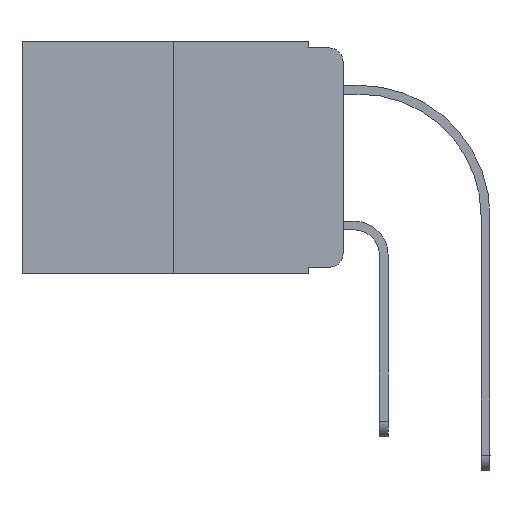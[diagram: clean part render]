
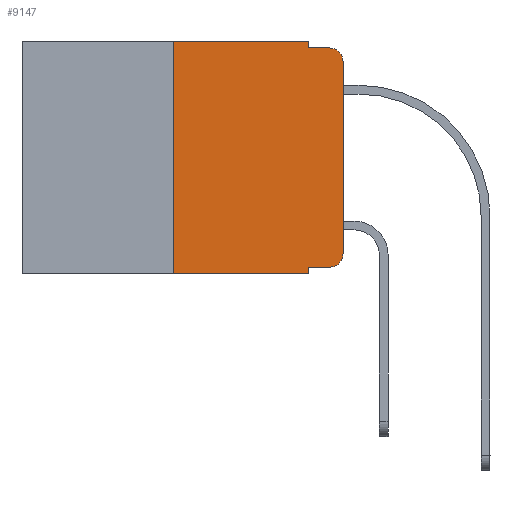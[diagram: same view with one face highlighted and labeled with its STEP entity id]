
A CAD part, left-side view. The second image highlights one B-rep face of the part: STEP entity #9147.
In plain terms, the highlighted planar face has unit normal (-1, 0, 0).
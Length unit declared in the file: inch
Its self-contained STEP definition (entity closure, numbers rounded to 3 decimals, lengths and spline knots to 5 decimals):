
#3 = DIRECTION ( 'NONE',  ( 0., 0., -1. ) ) ;
#83 = FACE_OUTER_BOUND ( 'NONE', #6889, .T. ) ;
#214 = CARTESIAN_POINT ( 'NONE',  ( 0., 0., -0.313 ) ) ;
#323 = ORIENTED_EDGE ( 'NONE', *, *, #11098, .T. ) ;
#342 = VERTEX_POINT ( 'NONE', #9852 ) ;
#380 = VERTEX_POINT ( 'NONE', #2476 ) ;
#1178 = CARTESIAN_POINT ( 'NONE',  ( 0., 0.051, 0. ) ) ;
#1305 = ORIENTED_EDGE ( 'NONE', *, *, #3405, .T. ) ;
#1357 = CARTESIAN_POINT ( 'NONE',  ( 0., 0.051, -0.01 ) ) ;
#2319 = CIRCLE ( 'NONE', #10659, 0.02 ) ;
#2476 = CARTESIAN_POINT ( 'NONE',  ( 0., 0., -0.03 ) ) ;
#2523 = DIRECTION ( 'NONE',  ( 0., -1., 0. ) ) ;
#2785 = VERTEX_POINT ( 'NONE', #7133 ) ;
#2890 = ORIENTED_EDGE ( 'NONE', *, *, #10798, .T. ) ;
#3113 = CARTESIAN_POINT ( 'NONE',  ( 0., 0.051, -0.333 ) ) ;
#3405 = EDGE_CURVE ( 'NONE', #9787, #10544, #13211, .T. ) ;
#3697 = VECTOR ( 'NONE', #7472, 39.37008 ) ;
#3719 = VECTOR ( 'NONE', #14480, 39.37008 ) ;
#3730 = VERTEX_POINT ( 'NONE', #1357 ) ;
#4233 = VECTOR ( 'NONE', #2523, 39.37008 ) ;
#4420 = ORIENTED_EDGE ( 'NONE', *, *, #8532, .F. ) ;
#4503 = EDGE_CURVE ( 'NONE', #342, #10544, #4986, .T. ) ;
#4505 = EDGE_CURVE ( 'NONE', #6124, #380, #13257, .T. ) ;
#4549 = VERTEX_POINT ( 'NONE', #7572 ) ;
#4603 = CARTESIAN_POINT ( 'NONE',  ( 0., 0.473, 0. ) ) ;
#4986 = LINE ( 'NONE', #9530, #6417 ) ;
#5717 = DIRECTION ( 'NONE',  ( -1., 0., 0. ) ) ;
#5748 = DIRECTION ( 'NONE',  ( 0., 0., -1. ) ) ;
#6090 = ORIENTED_EDGE ( 'NONE', *, *, #10879, .F. ) ;
#6124 = VERTEX_POINT ( 'NONE', #214 ) ;
#6183 = CARTESIAN_POINT ( 'NONE',  ( 0., 0.473, -0.343 ) ) ;
#6202 = DIRECTION ( 'NONE',  ( -1., 0., 0. ) ) ;
#6411 = CARTESIAN_POINT ( 'NONE',  ( 0., 0.051, -0.01 ) ) ;
#6417 = VECTOR ( 'NONE', #8397, 39.37008 ) ;
#6694 = PLANE ( 'NONE',  #13250 ) ;
#6889 = EDGE_LOOP ( 'NONE', ( #9362, #9451, #10519, #14582, #6090, #4420, #1305, #10464, #323, #2890 ) ) ;
#6958 = CARTESIAN_POINT ( 'NONE',  ( 0., 0.25, 0. ) ) ;
#7044 = AXIS2_PLACEMENT_3D ( 'NONE', #11820, #6202, #8303 ) ;
#7133 = CARTESIAN_POINT ( 'NONE',  ( 0., 0.02, -0.333 ) ) ;
#7251 = VERTEX_POINT ( 'NONE', #1178 ) ;
#7472 = DIRECTION ( 'NONE',  ( 0., 0., 1. ) ) ;
#7572 = CARTESIAN_POINT ( 'NONE',  ( 0., 0.02, -0.01 ) ) ;
#7638 = DIRECTION ( 'NONE',  ( 0., 0., 1. ) ) ;
#8252 = VECTOR ( 'NONE', #5748, 39.37008 ) ;
#8303 = DIRECTION ( 'NONE',  ( 0., 0., -1. ) ) ;
#8331 = VECTOR ( 'NONE', #7638, 39.37008 ) ;
#8377 = EDGE_CURVE ( 'NONE', #380, #4549, #13973, .T. ) ;
#8397 = DIRECTION ( 'NONE',  ( 0., 0., -1. ) ) ;
#8510 = VECTOR ( 'NONE', #13055, 39.37008 ) ;
#8532 = EDGE_CURVE ( 'NONE', #9787, #12848, #8795, .T. ) ;
#8705 = VECTOR ( 'NONE', #14181, 39.37008 ) ;
#8795 = LINE ( 'NONE', #10917, #3697 ) ;
#9072 = DIRECTION ( 'NONE',  ( 1., 0., 0. ) ) ;
#9147 = ADVANCED_FACE ( 'NONE', ( #83 ), #6694, .F. ) ;
#9362 = ORIENTED_EDGE ( 'NONE', *, *, #4505, .T. ) ;
#9369 = CARTESIAN_POINT ( 'NONE',  ( 0., 0.473, 0. ) ) ;
#9451 = ORIENTED_EDGE ( 'NONE', *, *, #8377, .T. ) ;
#9530 = CARTESIAN_POINT ( 'NONE',  ( 0., 0.051, 0. ) ) ;
#9787 = VERTEX_POINT ( 'NONE', #12968 ) ;
#9852 = CARTESIAN_POINT ( 'NONE',  ( 0., 0.051, -0.333 ) ) ;
#10002 = EDGE_CURVE ( 'NONE', #7251, #3730, #11423, .T. ) ;
#10464 = ORIENTED_EDGE ( 'NONE', *, *, #4503, .F. ) ;
#10519 = ORIENTED_EDGE ( 'NONE', *, *, #13519, .F. ) ;
#10544 = VERTEX_POINT ( 'NONE', #12986 ) ;
#10659 = AXIS2_PLACEMENT_3D ( 'NONE', #12521, #5717, #3 ) ;
#10798 = EDGE_CURVE ( 'NONE', #2785, #6124, #2319, .T. ) ;
#10879 = EDGE_CURVE ( 'NONE', #12848, #7251, #13928, .T. ) ;
#10917 = CARTESIAN_POINT ( 'NONE',  ( 0., 0.25, 0. ) ) ;
#11098 = EDGE_CURVE ( 'NONE', #342, #2785, #13332, .T. ) ;
#11423 = LINE ( 'NONE', #13819, #8252 ) ;
#11820 = CARTESIAN_POINT ( 'NONE',  ( 0., 0.02, -0.03 ) ) ;
#12361 = CARTESIAN_POINT ( 'NONE',  ( 0., 0., 0. ) ) ;
#12521 = CARTESIAN_POINT ( 'NONE',  ( 0., 0.02, -0.313 ) ) ;
#12848 = VERTEX_POINT ( 'NONE', #6958 ) ;
#12968 = CARTESIAN_POINT ( 'NONE',  ( 0., 0.25, -0.343 ) ) ;
#12986 = CARTESIAN_POINT ( 'NONE',  ( 0., 0.051, -0.343 ) ) ;
#13055 = DIRECTION ( 'NONE',  ( 0., -1., 0. ) ) ;
#13089 = LINE ( 'NONE', #6411, #3719 ) ;
#13211 = LINE ( 'NONE', #6183, #8705 ) ;
#13250 = AXIS2_PLACEMENT_3D ( 'NONE', #4603, #9072, #13643 ) ;
#13257 = LINE ( 'NONE', #12361, #8331 ) ;
#13332 = LINE ( 'NONE', #3113, #8510 ) ;
#13519 = EDGE_CURVE ( 'NONE', #3730, #4549, #13089, .T. ) ;
#13643 = DIRECTION ( 'NONE',  ( 0., 0., -1. ) ) ;
#13819 = CARTESIAN_POINT ( 'NONE',  ( 0., 0.051, 0. ) ) ;
#13928 = LINE ( 'NONE', #9369, #4233 ) ;
#13973 = CIRCLE ( 'NONE', #7044, 0.02 ) ;
#14181 = DIRECTION ( 'NONE',  ( 0., -1., 0. ) ) ;
#14480 = DIRECTION ( 'NONE',  ( 0., -1., 0. ) ) ;
#14582 = ORIENTED_EDGE ( 'NONE', *, *, #10002, .F. ) ;
